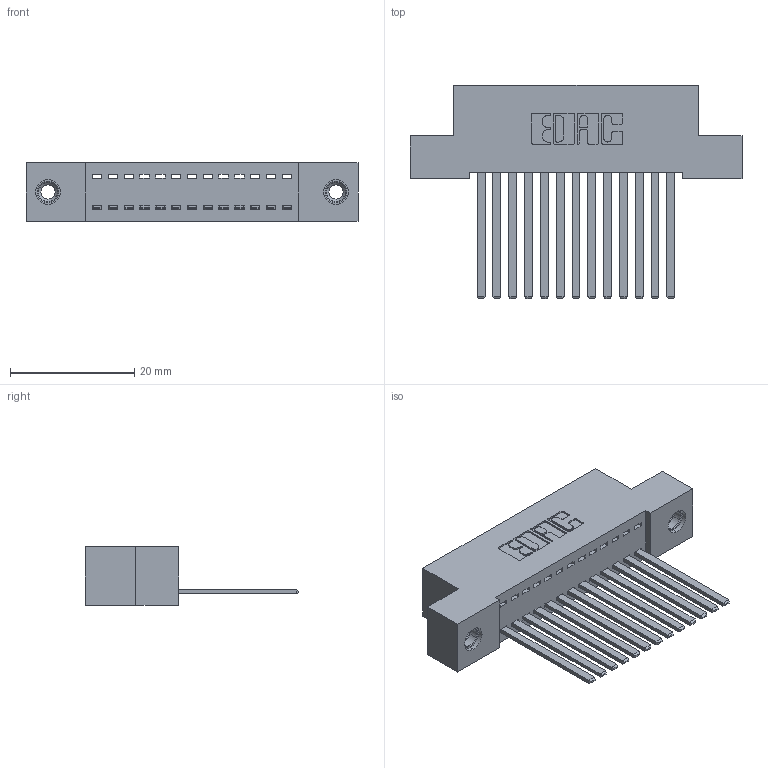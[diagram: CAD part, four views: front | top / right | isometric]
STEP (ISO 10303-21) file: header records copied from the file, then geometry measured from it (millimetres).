
FILE_DESCRIPTION (( 'STEP AP203' ), '1' );
FILE_NAME ('342-013-544-108.STEP', '2018-08-10T16:31:51', ( '' ), ( '' ), 'SwSTEP 2.0', 'SolidWorks 2016', '' );
FILE_SCHEMA (( 'CONFIG_CONTROL_DESIGN' ));
Length unit declared in the file: inch
Products named in the file (4): 345-250-001_345-250-003-102; 342-013-544-108; 342 Part_TI; 345-292-001_345-293-144
Assembly tree (16 placements, depth 2):
  342-013-544-108
    342 Part_TI
    345-292-001_345-293-144  x13
    345-250-001_345-250-003-102  x2
Bounding box: 53.34 x 34.3 x 9.4 mm (x, y, z)
Volume: 4714.9 mm3; surface area: 6828.5 mm2
Topology: 16 solids, 16 shells, 846 faces, 2489 edges, 1634 vertices
Faces by surface type: plane 592, cylinder 238, cone 12, torus 4
Entity records: 12568 total; most frequent: CARTESIAN_POINT 2152, ORIENTED_EDGE 2094, DIRECTION 1903, EDGE_CURVE 1047, VECTOR 903, LINE 903, VERTEX_POINT 692, AXIS2_PLACEMENT_3D 500
